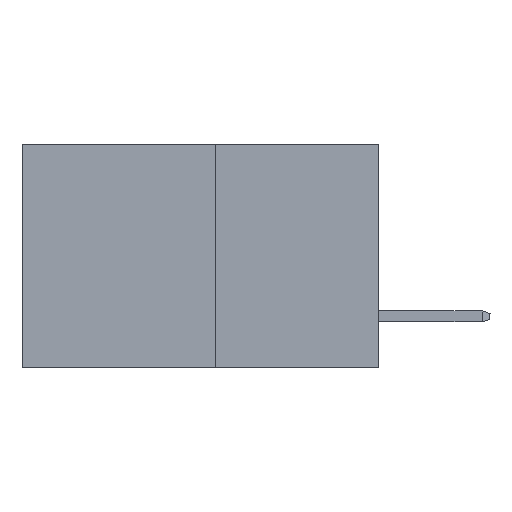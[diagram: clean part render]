
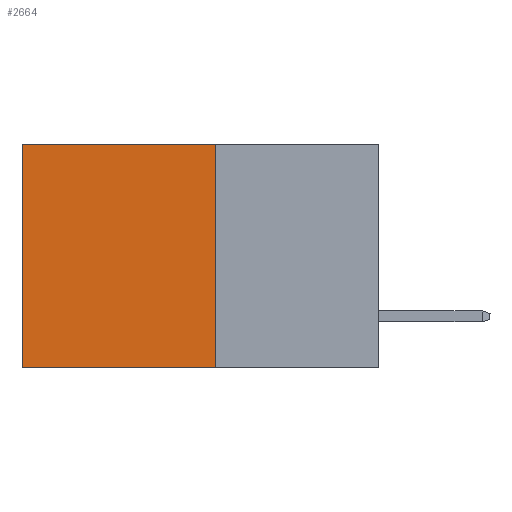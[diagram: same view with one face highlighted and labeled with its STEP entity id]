
A CAD part, left-side view. The second image highlights one B-rep face of the part: STEP entity #2664.
In plain terms, the highlighted planar face has unit normal (-1, 0, 0).
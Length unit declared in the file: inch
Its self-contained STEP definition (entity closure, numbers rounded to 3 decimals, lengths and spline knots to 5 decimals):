
#38 = CARTESIAN_POINT ( 'NONE',  ( 0.277, 0.59, 0. ) ) ;
#286 = EDGE_CURVE ( 'NONE', #5629, #10416, #8903, .T. ) ;
#915 = VECTOR ( 'NONE', #1097, 39.37008 ) ;
#1097 = DIRECTION ( 'NONE',  ( 0., 1., 0. ) ) ;
#1321 = VECTOR ( 'NONE', #3219, 39.37008 ) ;
#1507 = DIRECTION ( 'NONE',  ( 0., 0., -1. ) ) ;
#1508 = DIRECTION ( 'NONE',  ( 1., 0., 0. ) ) ;
#1625 = ORIENTED_EDGE ( 'NONE', *, *, #2748, .T. ) ;
#1933 = FACE_OUTER_BOUND ( 'NONE', #11535, .T. ) ;
#2024 = CARTESIAN_POINT ( 'NONE',  ( 0.277, 0.27, -0.37 ) ) ;
#2041 = DIRECTION ( 'NONE',  ( 0., 1., 0. ) ) ;
#2107 = CARTESIAN_POINT ( 'NONE',  ( 0.277, 0.27, 0. ) ) ;
#2411 = PLANE ( 'NONE',  #5906 ) ;
#2421 = CARTESIAN_POINT ( 'NONE',  ( 0.277, 0.27, -0.37 ) ) ;
#2664 = ADVANCED_FACE ( 'NONE', ( #1933 ), #2411, .F. ) ;
#2748 = EDGE_CURVE ( 'NONE', #4554, #5629, #4034, .T. ) ;
#2880 = EDGE_CURVE ( 'NONE', #9845, #10416, #12586, .T. ) ;
#3025 = CARTESIAN_POINT ( 'NONE',  ( 0.277, 0.59, -0.37 ) ) ;
#3219 = DIRECTION ( 'NONE',  ( 0., 0., -1. ) ) ;
#4034 = LINE ( 'NONE', #2107, #915 ) ;
#4291 = ORIENTED_EDGE ( 'NONE', *, *, #2880, .F. ) ;
#4554 = VERTEX_POINT ( 'NONE', #9695 ) ;
#4558 = CARTESIAN_POINT ( 'NONE',  ( 0.277, 0.27, -0.37 ) ) ;
#5629 = VERTEX_POINT ( 'NONE', #38 ) ;
#5707 = EDGE_CURVE ( 'NONE', #4554, #9845, #6104, .T. ) ;
#5906 = AXIS2_PLACEMENT_3D ( 'NONE', #2421, #1508, #1507 ) ;
#6104 = LINE ( 'NONE', #10038, #8065 ) ;
#6247 = ORIENTED_EDGE ( 'NONE', *, *, #286, .T. ) ;
#8065 = VECTOR ( 'NONE', #10304, 39.37008 ) ;
#8103 = ORIENTED_EDGE ( 'NONE', *, *, #5707, .F. ) ;
#8903 = LINE ( 'NONE', #3025, #1321 ) ;
#9695 = CARTESIAN_POINT ( 'NONE',  ( 0.277, 0.27, 0. ) ) ;
#9845 = VERTEX_POINT ( 'NONE', #4558 ) ;
#10038 = CARTESIAN_POINT ( 'NONE',  ( 0.277, 0.27, -0.37 ) ) ;
#10304 = DIRECTION ( 'NONE',  ( 0., 0., -1. ) ) ;
#10416 = VERTEX_POINT ( 'NONE', #12130 ) ;
#11535 = EDGE_LOOP ( 'NONE', ( #6247, #4291, #8103, #1625 ) ) ;
#12130 = CARTESIAN_POINT ( 'NONE',  ( 0.277, 0.59, -0.37 ) ) ;
#12303 = VECTOR ( 'NONE', #2041, 39.37008 ) ;
#12586 = LINE ( 'NONE', #2024, #12303 ) ;
